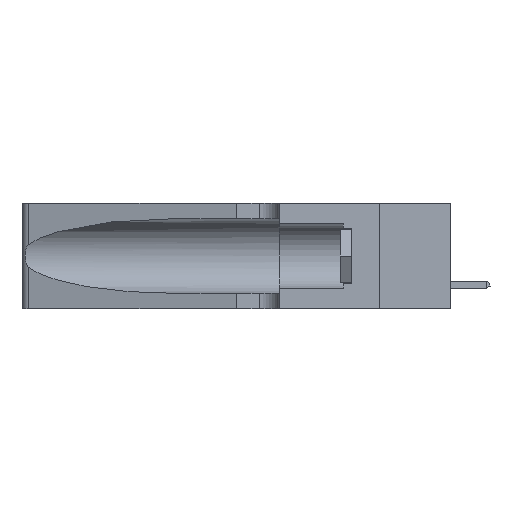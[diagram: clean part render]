
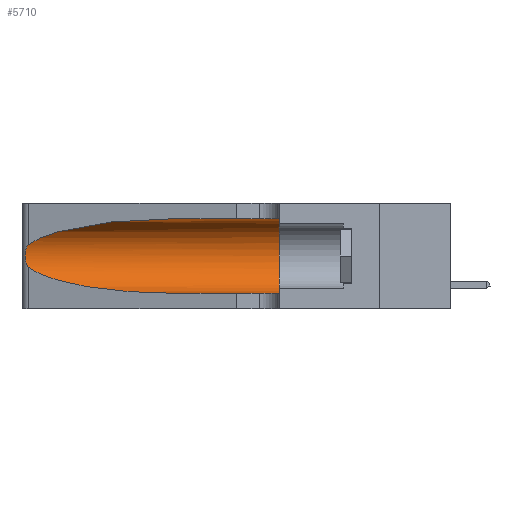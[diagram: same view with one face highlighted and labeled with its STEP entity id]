
A CAD part, left-side view. The second image highlights one B-rep face of the part: STEP entity #5710.
In plain terms, the highlighted cylindrical face has radius 3.308 mm (diameter 6.617 mm), a partial arc.
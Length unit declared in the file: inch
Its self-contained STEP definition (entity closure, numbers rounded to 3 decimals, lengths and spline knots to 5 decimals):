
#219 = CARTESIAN_POINT ( 'NONE',  ( 0.1305, 1.61858, 0.185 ) ) ;
#322 = DIRECTION ( 'NONE',  ( 0., 0., -1. ) ) ;
#491 = CARTESIAN_POINT ( 'NONE',  ( 0.1305, 0.35, 0.185 ) ) ;
#629 = DIRECTION ( 'NONE',  ( 0., -1., 0. ) ) ;
#1555 = VECTOR ( 'NONE', #17381, 39.37008 ) ;
#1744 = B_SPLINE_CURVE_WITH_KNOTS ( 'NONE', 3,
 ( #15106, #9619, #33693, #33452, #30908, #17797, #23007, #17686, #17554, #33336, #33578, #7038, #7159, #25818 ),
 .UNSPECIFIED., .F., .F.,
 ( 4, 2, 2, 2, 2, 2, 4 ),
 ( 0., 0.00027, 0.00053, 0.00107, 0.0016, 0.00187, 0.00214 ),
 .UNSPECIFIED. ) ;
#1887 = CARTESIAN_POINT ( 'NONE',  ( 0.1305, 0.72297, 0.31525 ) ) ;
#2948 = CARTESIAN_POINT ( 'NONE',  ( 0.18966, 0.96281, 0.05475 ) ) ;
#3182 = CARTESIAN_POINT ( 'NONE',  ( 0.1305, 1.61858, 0.05475 ) ) ;
#3975 = CARTESIAN_POINT ( 'NONE',  ( 0.1305, 1.61858, 0.31525 ) ) ;
#4538 = CARTESIAN_POINT ( 'NONE',  ( 0.2373, 1.15595, 0.28018 ) ) ;
#5710 = ADVANCED_FACE ( 'NONE', ( #21762 ), #7611, .F. ) ;
#6036 = ORIENTED_EDGE ( 'NONE', *, *, #20597, .T. ) ;
#7038 = CARTESIAN_POINT ( 'NONE',  ( 0.25639, 1.23186, 0.15144 ) ) ;
#7159 = CARTESIAN_POINT ( 'NONE',  ( 0.25555, 1.22993, 0.14849 ) ) ;
#7611 = CYLINDRICAL_SURFACE ( 'NONE', #15910, 0.13025 ) ;
#8092 = CIRCLE ( 'NONE', #30131, 0.13025 ) ;
#8196 = DIRECTION ( 'NONE',  ( 0., -1., 0. ) ) ;
#8242 = EDGE_CURVE ( 'NONE', #17689, #25655, #32723, .T. ) ;
#8864 = VECTOR ( 'NONE', #629, 39.37008 ) ;
#9510 = VERTEX_POINT ( 'NONE', #26237 ) ;
#9619 = CARTESIAN_POINT ( 'NONE',  ( 0.25555, 1.22994, 0.2215 ) ) ;
#10433 = ORIENTED_EDGE ( 'NONE', *, *, #34252, .T. ) ;
#10954 = CARTESIAN_POINT ( 'NONE',  ( 0.2373, 1.15595, 0.08982 ) ) ;
#11416 = CARTESIAN_POINT ( 'NONE',  ( 0.25487, 1.22718, 0.14631 ) ) ;
#12273 = CARTESIAN_POINT ( 'NONE',  ( 0.25487, 1.22718, 0.22369 ) ) ;
#12879 = CARTESIAN_POINT ( 'NONE',  ( 0.1305, 0.35, 0.05475 ) ) ;
#13922 = VERTEX_POINT ( 'NONE', #12273 ) ;
#15106 = CARTESIAN_POINT ( 'NONE',  ( 0.25487, 1.22718, 0.22369 ) ) ;
#15910 = AXIS2_PLACEMENT_3D ( 'NONE', #219, #8196, #322 ) ;
#16317 = CARTESIAN_POINT ( 'NONE',  ( 0.1305, 0.72297, 0.05475 ) ) ;
#16458 = CARTESIAN_POINT ( 'NONE',  ( 0.1305, 0.72297, 0.31525 ) ) ;
#17010 = EDGE_CURVE ( 'NONE', #25655, #29433, #8092, .T. ) ;
#17238 = LINE ( 'NONE', #3182, #8864 ) ;
#17381 = DIRECTION ( 'NONE',  ( 0., -1., 0. ) ) ;
#17554 = CARTESIAN_POINT ( 'NONE',  ( 0.26017, 1.23833, 0.17102 ) ) ;
#17686 = CARTESIAN_POINT ( 'NONE',  ( 0.26075, 1.23896, 0.178 ) ) ;
#17689 = VERTEX_POINT ( 'NONE', #16458 ) ;
#17797 = CARTESIAN_POINT ( 'NONE',  ( 0.26018, 1.23835, 0.19895 ) ) ;
#18217 = ORIENTED_EDGE ( 'NONE', *, *, #20396, .T. ) ;
#18683 = ORIENTED_EDGE ( 'NONE', *, *, #17010, .F. ) ;
#19558 = CARTESIAN_POINT ( 'NONE',  ( 0.1305, 0.72297, 0.05475 ) ) ;
#19851 = EDGE_LOOP ( 'NONE', ( #18217, #19937, #10433, #6036, #18683, #33607 ) ) ;
#19937 = ORIENTED_EDGE ( 'NONE', *, *, #24055, .T. ) ;
#20396 = EDGE_CURVE ( 'NONE', #17689, #13922, #25430, .T. ) ;
#20597 = EDGE_CURVE ( 'NONE', #22136, #29433, #17238, .T. ) ;
#20923 = CARTESIAN_POINT ( 'NONE',  ( 0.1305, 0.35, 0.31525 ) ) ;
#21760 = DIRECTION ( 'NONE',  ( 0., 1., 0. ) ) ;
#21762 = FACE_OUTER_BOUND ( 'NONE', #19851, .T. ) ;
#22136 = VERTEX_POINT ( 'NONE', #19558 ) ;
#22331 = DIRECTION ( 'NONE',  ( 0., 0., 1. ) ) ;
#23007 = CARTESIAN_POINT ( 'NONE',  ( 0.26075, 1.23896, 0.19203 ) ) ;
#24055 = EDGE_CURVE ( 'NONE', #13922, #9510, #1744, .T. ) ;
#25430 =( BOUNDED_CURVE ( )  B_SPLINE_CURVE ( 3, ( #1887, #33840, #4538, #28511 ),
 .UNSPECIFIED., .F., .F. ) 
 B_SPLINE_CURVE_WITH_KNOTS ( ( 4, 4 ),
 ( 1.5708, 2.84003 ),
 .UNSPECIFIED. ) 
 CURVE ( )  GEOMETRIC_REPRESENTATION_ITEM ( )  RATIONAL_B_SPLINE_CURVE ( ( 1., 0.87, 0.87, 1. ) ) 
 REPRESENTATION_ITEM ( '' )  );
#25655 = VERTEX_POINT ( 'NONE', #20923 ) ;
#25818 = CARTESIAN_POINT ( 'NONE',  ( 0.25487, 1.22718, 0.14631 ) ) ;
#26237 = CARTESIAN_POINT ( 'NONE',  ( 0.25487, 1.22718, 0.14631 ) ) ;
#26869 =( BOUNDED_CURVE ( )  B_SPLINE_CURVE ( 3, ( #11416, #10954, #2948, #16317 ),
 .UNSPECIFIED., .F., .F. ) 
 B_SPLINE_CURVE_WITH_KNOTS ( ( 4, 4 ),
 ( 3.44316, 4.71239 ),
 .UNSPECIFIED. ) 
 CURVE ( )  GEOMETRIC_REPRESENTATION_ITEM ( )  RATIONAL_B_SPLINE_CURVE ( ( 1., 0.87, 0.87, 1. ) ) 
 REPRESENTATION_ITEM ( '' )  );
#28511 = CARTESIAN_POINT ( 'NONE',  ( 0.25487, 1.22718, 0.22369 ) ) ;
#29433 = VERTEX_POINT ( 'NONE', #12879 ) ;
#30131 = AXIS2_PLACEMENT_3D ( 'NONE', #491, #21760, #22331 ) ;
#30908 = CARTESIAN_POINT ( 'NONE',  ( 0.25854, 1.2359, 0.20912 ) ) ;
#32723 = LINE ( 'NONE', #3975, #1555 ) ;
#33336 = CARTESIAN_POINT ( 'NONE',  ( 0.25856, 1.23593, 0.16098 ) ) ;
#33452 = CARTESIAN_POINT ( 'NONE',  ( 0.25787, 1.23484, 0.2124 ) ) ;
#33578 = CARTESIAN_POINT ( 'NONE',  ( 0.25789, 1.23486, 0.15765 ) ) ;
#33607 = ORIENTED_EDGE ( 'NONE', *, *, #8242, .F. ) ;
#33693 = CARTESIAN_POINT ( 'NONE',  ( 0.25639, 1.23184, 0.21858 ) ) ;
#33840 = CARTESIAN_POINT ( 'NONE',  ( 0.18966, 0.96281, 0.31525 ) ) ;
#34252 = EDGE_CURVE ( 'NONE', #9510, #22136, #26869, .T. ) ;
